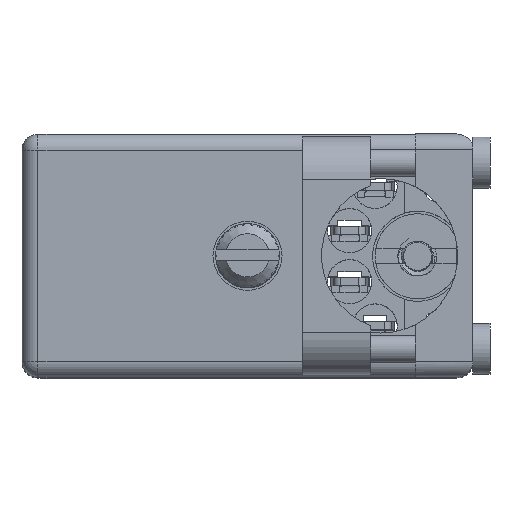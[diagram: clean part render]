
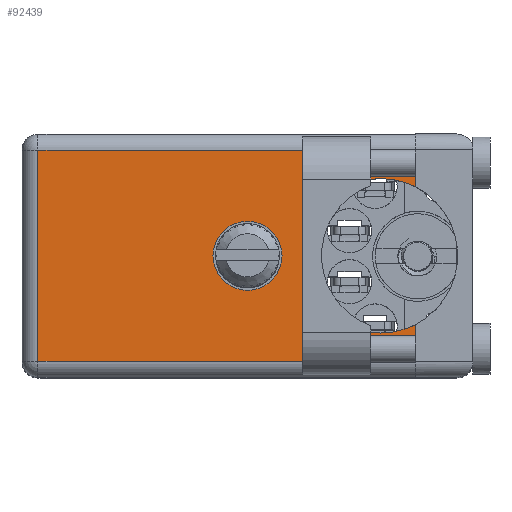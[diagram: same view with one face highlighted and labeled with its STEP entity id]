
A CAD part, top view. The second image highlights one B-rep face of the part: STEP entity #92439.
In plain terms, the highlighted face is planar.
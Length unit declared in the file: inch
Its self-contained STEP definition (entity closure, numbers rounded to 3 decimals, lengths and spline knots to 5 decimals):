
#2797 = CARTESIAN_POINT ( 'NONE',  ( -0.6625, 0.806, -0.3105 ) ) ;
#8501 = DIRECTION ( 'NONE',  ( -1., 0., 0. ) ) ;
#8535 = VECTOR ( 'NONE', #131936, 39.37008 ) ;
#10150 = CARTESIAN_POINT ( 'NONE',  ( 0.4925, 0.806, 0.3575 ) ) ;
#11363 = CIRCLE ( 'NONE', #96536, 0.227 ) ;
#12114 = EDGE_CURVE ( 'NONE', #124062, #127269, #91498, .T. ) ;
#15256 = EDGE_CURVE ( 'NONE', #141478, #176471, #11363, .T. ) ;
#16604 = ORIENTED_EDGE ( 'NONE', *, *, #159421, .F. ) ;
#17552 = DIRECTION ( 'NONE',  ( 0., 1., 0. ) ) ;
#19585 = CARTESIAN_POINT ( 'NONE',  ( 0.4925, 0.806, 0.3575 ) ) ;
#27945 = VERTEX_POINT ( 'NONE', #83679 ) ;
#31850 = EDGE_LOOP ( 'NONE', ( #36962, #172093, #69297, #170187, #120505, #16604, #36337, #66699 ) ) ;
#32670 = CARTESIAN_POINT ( 'NONE',  ( -0.6625, 0.806, -0.3575 ) ) ;
#34390 = DIRECTION ( 'NONE',  ( 0., 1., 0. ) ) ;
#35134 = CIRCLE ( 'NONE', #146490, 0.1015 ) ;
#36337 = ORIENTED_EDGE ( 'NONE', *, *, #87372, .F. ) ;
#36748 = VERTEX_POINT ( 'NONE', #88392 ) ;
#36962 = ORIENTED_EDGE ( 'NONE', *, *, #79345, .F. ) ;
#39720 = CARTESIAN_POINT ( 'NONE',  ( -0.6155, 0.806, 0.3105 ) ) ;
#43481 = VERTEX_POINT ( 'NONE', #64155 ) ;
#50824 = VECTOR ( 'NONE', #147142, 39.37008 ) ;
#63358 = DIRECTION ( 'NONE',  ( -1., 0., 0. ) ) ;
#63717 = PLANE ( 'NONE',  #166196 ) ;
#64155 = CARTESIAN_POINT ( 'NONE',  ( 0., 0.806, 0.1015 ) ) ;
#66699 = ORIENTED_EDGE ( 'NONE', *, *, #15256, .F. ) ;
#69297 = ORIENTED_EDGE ( 'NONE', *, *, #188609, .T. ) ;
#72556 = VERTEX_POINT ( 'NONE', #172747 ) ;
#78235 = CARTESIAN_POINT ( 'NONE',  ( 0., 0.806, 0. ) ) ;
#78814 = CARTESIAN_POINT ( 'NONE',  ( 0.3905, 0.806, 0. ) ) ;
#79345 = EDGE_CURVE ( 'NONE', #124062, #141478, #131314, .T. ) ;
#80540 = DIRECTION ( 'NONE',  ( -1., 0., 0. ) ) ;
#82151 = LINE ( 'NONE', #147809, #50824 ) ;
#83679 = CARTESIAN_POINT ( 'NONE',  ( 0., 0.806, -0.1015 ) ) ;
#85450 = CIRCLE ( 'NONE', #196422, 0.1015 ) ;
#85824 = EDGE_CURVE ( 'NONE', #136136, #36748, #82151, .T. ) ;
#87372 = EDGE_CURVE ( 'NONE', #176471, #135010, #89093, .T. ) ;
#88392 = CARTESIAN_POINT ( 'NONE',  ( 0.4925, 0.806, 0.3105 ) ) ;
#89093 = CIRCLE ( 'NONE', #148624, 0.227 ) ;
#91498 = LINE ( 'NONE', #2797, #134708 ) ;
#92439 = ADVANCED_FACE ( 'NONE', ( #165557, #148809 ), #63717, .T. ) ;
#96536 = AXIS2_PLACEMENT_3D ( 'NONE', #175448, #188952, #99440 ) ;
#96902 = CARTESIAN_POINT ( 'NONE',  ( 0.3905, 0.806, 0.227 ) ) ;
#97582 = CIRCLE ( 'NONE', #105300, 0.227 ) ;
#98330 = EDGE_CURVE ( 'NONE', #43481, #27945, #35134, .T. ) ;
#99440 = DIRECTION ( 'NONE',  ( -1., 0., 0. ) ) ;
#103200 = DIRECTION ( 'NONE',  ( 0., 0., 1. ) ) ;
#105300 = AXIS2_PLACEMENT_3D ( 'NONE', #138012, #139352, #108382 ) ;
#108382 = DIRECTION ( 'NONE',  ( -1., 0., 0. ) ) ;
#108449 = VECTOR ( 'NONE', #110423, 39.37008 ) ;
#110423 = DIRECTION ( 'NONE',  ( 0., 0., 1. ) ) ;
#113235 = VECTOR ( 'NONE', #103200, 39.37008 ) ;
#116275 = ORIENTED_EDGE ( 'NONE', *, *, #191058, .F. ) ;
#120009 = EDGE_CURVE ( 'NONE', #72556, #36748, #156499, .T. ) ;
#120505 = ORIENTED_EDGE ( 'NONE', *, *, #120009, .F. ) ;
#124062 = VERTEX_POINT ( 'NONE', #152157 ) ;
#127269 = VERTEX_POINT ( 'NONE', #129870 ) ;
#129251 = DIRECTION ( 'NONE',  ( 0., 0., 1. ) ) ;
#129870 = CARTESIAN_POINT ( 'NONE',  ( -0.6155, 0.806, -0.3105 ) ) ;
#131314 = LINE ( 'NONE', #10150, #8535 ) ;
#131936 = DIRECTION ( 'NONE',  ( 0., 0., 1. ) ) ;
#134708 = VECTOR ( 'NONE', #8501, 39.37008 ) ;
#134992 = DIRECTION ( 'NONE',  ( 0., 1., 0. ) ) ;
#135010 = VERTEX_POINT ( 'NONE', #96902 ) ;
#136136 = VERTEX_POINT ( 'NONE', #39720 ) ;
#138012 = CARTESIAN_POINT ( 'NONE',  ( 0.3905, 0.806, 0. ) ) ;
#139352 = DIRECTION ( 'NONE',  ( 0., 1., 0. ) ) ;
#141478 = VERTEX_POINT ( 'NONE', #198827 ) ;
#145838 = ORIENTED_EDGE ( 'NONE', *, *, #98330, .F. ) ;
#146490 = AXIS2_PLACEMENT_3D ( 'NONE', #78235, #34390, #129251 ) ;
#147142 = DIRECTION ( 'NONE',  ( 1., 0., 0. ) ) ;
#147809 = CARTESIAN_POINT ( 'NONE',  ( 0.4925, 0.806, 0.3105 ) ) ;
#147847 = DIRECTION ( 'NONE',  ( 0., 0., 1. ) ) ;
#148624 = AXIS2_PLACEMENT_3D ( 'NONE', #78814, #17552, #63358 ) ;
#148809 = FACE_BOUND ( 'NONE', #167291, .T. ) ;
#150478 = CARTESIAN_POINT ( 'NONE',  ( 0., 0.806, 0. ) ) ;
#152157 = CARTESIAN_POINT ( 'NONE',  ( 0.4925, 0.806, -0.3105 ) ) ;
#154120 = LINE ( 'NONE', #195364, #113235 ) ;
#156499 = LINE ( 'NONE', #19585, #108449 ) ;
#159421 = EDGE_CURVE ( 'NONE', #135010, #72556, #97582, .T. ) ;
#165557 = FACE_OUTER_BOUND ( 'NONE', #31850, .T. ) ;
#166196 = AXIS2_PLACEMENT_3D ( 'NONE', #32670, #171308, #80540 ) ;
#167291 = EDGE_LOOP ( 'NONE', ( #145838, #116275 ) ) ;
#170187 = ORIENTED_EDGE ( 'NONE', *, *, #85824, .T. ) ;
#171308 = DIRECTION ( 'NONE',  ( 0., 1., 0. ) ) ;
#172093 = ORIENTED_EDGE ( 'NONE', *, *, #12114, .T. ) ;
#172747 = CARTESIAN_POINT ( 'NONE',  ( 0.4925, 0.806, 0.20279 ) ) ;
#175448 = CARTESIAN_POINT ( 'NONE',  ( 0.3905, 0.806, 0. ) ) ;
#176471 = VERTEX_POINT ( 'NONE', #193587 ) ;
#188609 = EDGE_CURVE ( 'NONE', #127269, #136136, #154120, .T. ) ;
#188952 = DIRECTION ( 'NONE',  ( 0., 1., 0. ) ) ;
#191058 = EDGE_CURVE ( 'NONE', #27945, #43481, #85450, .T. ) ;
#193587 = CARTESIAN_POINT ( 'NONE',  ( 0.3905, 0.806, -0.227 ) ) ;
#195364 = CARTESIAN_POINT ( 'NONE',  ( -0.6155, 0.806, -0.3575 ) ) ;
#196422 = AXIS2_PLACEMENT_3D ( 'NONE', #150478, #134992, #147847 ) ;
#198827 = CARTESIAN_POINT ( 'NONE',  ( 0.4925, 0.806, -0.20279 ) ) ;
